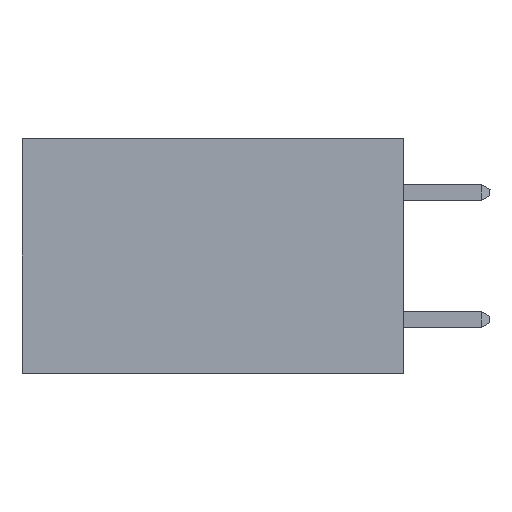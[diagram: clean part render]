
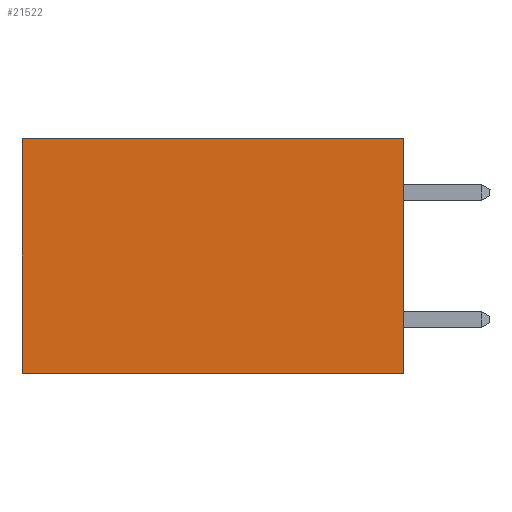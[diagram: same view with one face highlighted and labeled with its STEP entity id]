
A CAD part, left-side view. The second image highlights one B-rep face of the part: STEP entity #21522.
In plain terms, the highlighted planar face has unit normal (-1, 0, 0).
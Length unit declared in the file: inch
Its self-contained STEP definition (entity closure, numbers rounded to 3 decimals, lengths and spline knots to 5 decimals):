
#828 = CARTESIAN_POINT ( 'NONE',  ( 0.2875, 0.6, 0. ) ) ;
#1329 = EDGE_CURVE ( 'NONE', #33944, #28508, #20333, .T. ) ;
#3383 = DIRECTION ( 'NONE',  ( 0., 0., -1. ) ) ;
#4391 = DIRECTION ( 'NONE',  ( 0., 1., 0. ) ) ;
#5431 = EDGE_CURVE ( 'NONE', #28508, #22399, #39795, .T. ) ;
#8260 = ORIENTED_EDGE ( 'NONE', *, *, #27843, .F. ) ;
#8305 = LINE ( 'NONE', #25768, #20421 ) ;
#9798 = DIRECTION ( 'NONE',  ( 0., 0., -1. ) ) ;
#9956 = VECTOR ( 'NONE', #3383, 39.37008 ) ;
#15152 = CARTESIAN_POINT ( 'NONE',  ( 0.2875, 0., -0.37 ) ) ;
#15196 = ORIENTED_EDGE ( 'NONE', *, *, #5431, .T. ) ;
#18181 = EDGE_LOOP ( 'NONE', ( #15196, #30995, #8260, #21041 ) ) ;
#18799 = DIRECTION ( 'NONE',  ( 0., 0., -1. ) ) ;
#20115 = PLANE ( 'NONE',  #26538 ) ;
#20276 = DIRECTION ( 'NONE',  ( 1., 0., 0. ) ) ;
#20333 = LINE ( 'NONE', #33170, #27463 ) ;
#20421 = VECTOR ( 'NONE', #9798, 39.37008 ) ;
#21041 = ORIENTED_EDGE ( 'NONE', *, *, #1329, .T. ) ;
#21522 = ADVANCED_FACE ( 'NONE', ( #34430 ), #20115, .F. ) ;
#21889 = CARTESIAN_POINT ( 'NONE',  ( 0.2875, 0., -0.37 ) ) ;
#22128 = CARTESIAN_POINT ( 'NONE',  ( 0.2875, 0.6, -0.37 ) ) ;
#22399 = VERTEX_POINT ( 'NONE', #22128 ) ;
#23369 = CARTESIAN_POINT ( 'NONE',  ( 0.2875, 0., 0. ) ) ;
#24863 = EDGE_CURVE ( 'NONE', #41062, #22399, #31816, .T. ) ;
#25768 = CARTESIAN_POINT ( 'NONE',  ( 0.2875, 0., 0. ) ) ;
#26538 = AXIS2_PLACEMENT_3D ( 'NONE', #23369, #20276, #18799 ) ;
#27463 = VECTOR ( 'NONE', #4391, 39.37008 ) ;
#27843 = EDGE_CURVE ( 'NONE', #33944, #41062, #8305, .T. ) ;
#28508 = VERTEX_POINT ( 'NONE', #828 ) ;
#30995 = ORIENTED_EDGE ( 'NONE', *, *, #24863, .F. ) ;
#31816 = LINE ( 'NONE', #21889, #36918 ) ;
#32431 = CARTESIAN_POINT ( 'NONE',  ( 0.2875, 0.6, 0. ) ) ;
#33170 = CARTESIAN_POINT ( 'NONE',  ( 0.2875, 0., 0. ) ) ;
#33944 = VERTEX_POINT ( 'NONE', #35599 ) ;
#34430 = FACE_OUTER_BOUND ( 'NONE', #18181, .T. ) ;
#35599 = CARTESIAN_POINT ( 'NONE',  ( 0.2875, 0., 0. ) ) ;
#35856 = DIRECTION ( 'NONE',  ( 0., 1., 0. ) ) ;
#36918 = VECTOR ( 'NONE', #35856, 39.37008 ) ;
#39795 = LINE ( 'NONE', #32431, #9956 ) ;
#41062 = VERTEX_POINT ( 'NONE', #15152 ) ;
